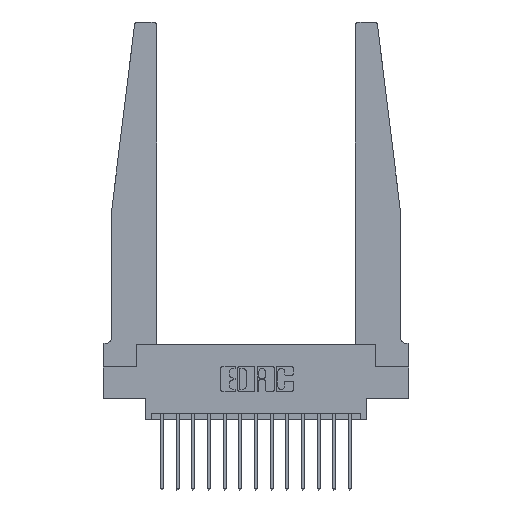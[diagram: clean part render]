
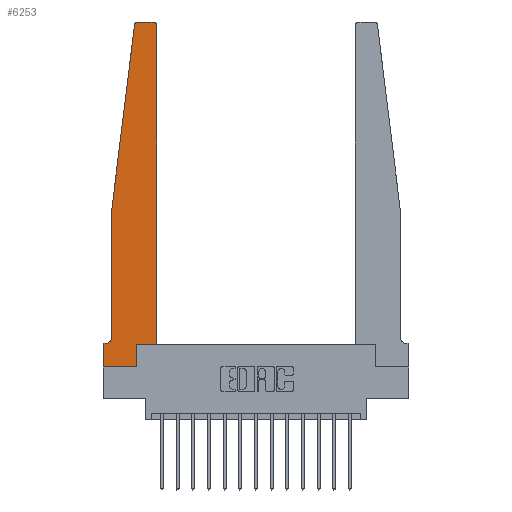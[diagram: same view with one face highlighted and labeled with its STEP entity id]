
A CAD part, top view. The second image highlights one B-rep face of the part: STEP entity #6253.
In plain terms, the highlighted planar face has unit normal (0, 0, 1).
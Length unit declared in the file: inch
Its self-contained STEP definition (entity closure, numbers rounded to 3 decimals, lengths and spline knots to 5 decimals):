
#14 = ORIENTED_EDGE ( 'NONE', *, *, #17315, .T. ) ;
#188 = LINE ( 'NONE', #2962, #15309 ) ;
#430 = CARTESIAN_POINT ( 'NONE',  ( 0.2605, 0.18, 0.37 ) ) ;
#870 = VECTOR ( 'NONE', #1512, 39.37008 ) ;
#922 = ORIENTED_EDGE ( 'NONE', *, *, #9882, .T. ) ;
#1371 = DIRECTION ( 'NONE',  ( 0., -1., 0. ) ) ;
#1512 = DIRECTION ( 'NONE',  ( 0., 1., 0. ) ) ;
#1520 = VECTOR ( 'NONE', #2605, 39.37008 ) ;
#1620 = FACE_OUTER_BOUND ( 'NONE', #4993, .T. ) ;
#2082 = CARTESIAN_POINT ( 'NONE',  ( 0.27653, 2.72, 0.37 ) ) ;
#2123 = DIRECTION ( 'NONE',  ( 0., 0., 1. ) ) ;
#2340 = VERTEX_POINT ( 'NONE', #15075 ) ;
#2605 = DIRECTION ( 'NONE',  ( 0., 1., 0. ) ) ;
#2628 = LINE ( 'NONE', #13582, #12087 ) ;
#2693 = LINE ( 'NONE', #5117, #1520 ) ;
#2732 = LINE ( 'NONE', #6477, #10902 ) ;
#2768 = VECTOR ( 'NONE', #9583, 39.37008 ) ;
#2829 = AXIS2_PLACEMENT_3D ( 'NONE', #16928, #10074, #8721 ) ;
#2962 = CARTESIAN_POINT ( 'NONE',  ( 0., 0., 0.37 ) ) ;
#2967 = DIRECTION ( 'NONE',  ( 0., 0., 1. ) ) ;
#3551 = EDGE_CURVE ( 'NONE', #14291, #2340, #7639, .T. ) ;
#3645 = ORIENTED_EDGE ( 'NONE', *, *, #12383, .T. ) ;
#3940 = ORIENTED_EDGE ( 'NONE', *, *, #3551, .T. ) ;
#4198 = LINE ( 'NONE', #430, #870 ) ;
#4570 = CARTESIAN_POINT ( 'NONE',  ( 0.24675, 2.72367, 0.37 ) ) ;
#4993 = EDGE_LOOP ( 'NONE', ( #14090, #14, #15382, #5123, #12599, #12041, #3645, #7133, #8450, #922, #17621, #3940 ) ) ;
#5117 = CARTESIAN_POINT ( 'NONE',  ( 0.425, 0.18, 0.37 ) ) ;
#5123 = ORIENTED_EDGE ( 'NONE', *, *, #12833, .T. ) ;
#5259 = VECTOR ( 'NONE', #12888, 39.37008 ) ;
#5308 = CARTESIAN_POINT ( 'NONE',  ( 0.425, 0.18, 0.37 ) ) ;
#5365 = VERTEX_POINT ( 'NONE', #8385 ) ;
#5480 = CARTESIAN_POINT ( 'NONE',  ( 0., 0.1875, 0.37 ) ) ;
#5982 = EDGE_CURVE ( 'NONE', #5365, #13628, #11136, .T. ) ;
#5983 = DIRECTION ( 'NONE',  ( -1., 0., 0. ) ) ;
#6066 = CARTESIAN_POINT ( 'NONE',  ( 0.065, 0.1875, 0.37 ) ) ;
#6074 = VERTEX_POINT ( 'NONE', #9248 ) ;
#6253 = ADVANCED_FACE ( 'NONE', ( #1620 ), #8157, .T. ) ;
#6271 = DIRECTION ( 'NONE',  ( 0., 0., 1. ) ) ;
#6477 = CARTESIAN_POINT ( 'NONE',  ( 0., 0., 0.37 ) ) ;
#6504 = AXIS2_PLACEMENT_3D ( 'NONE', #16967, #2123, #14427 ) ;
#7105 = CARTESIAN_POINT ( 'NONE',  ( 0.27653, 2.75, 0.37 ) ) ;
#7133 = ORIENTED_EDGE ( 'NONE', *, *, #14382, .T. ) ;
#7639 = CIRCLE ( 'NONE', #6504, 0.03 ) ;
#7668 = EDGE_CURVE ( 'NONE', #6074, #14740, #4198, .T. ) ;
#8157 = PLANE ( 'NONE',  #16912 ) ;
#8198 = EDGE_CURVE ( 'NONE', #13628, #11796, #8597, .T. ) ;
#8337 = CARTESIAN_POINT ( 'NONE',  ( 0.425, 2.72, 0.37 ) ) ;
#8339 = AXIS2_PLACEMENT_3D ( 'NONE', #2082, #6271, #17086 ) ;
#8385 = CARTESIAN_POINT ( 'NONE',  ( 0.065, 0.2375, 0.37 ) ) ;
#8422 = DIRECTION ( 'NONE',  ( 1., 0., 0. ) ) ;
#8450 = ORIENTED_EDGE ( 'NONE', *, *, #7668, .T. ) ;
#8541 = EDGE_CURVE ( 'NONE', #2340, #10288, #14152, .T. ) ;
#8597 = LINE ( 'NONE', #6066, #14146 ) ;
#8721 = DIRECTION ( 'NONE',  ( -1., 0., 0. ) ) ;
#8753 = CARTESIAN_POINT ( 'NONE',  ( 0.2605, 0.18, 0.37 ) ) ;
#9248 = CARTESIAN_POINT ( 'NONE',  ( 0.2605, 0., 0.37 ) ) ;
#9276 = DIRECTION ( 'NONE',  ( 0., -1., 0. ) ) ;
#9495 = VERTEX_POINT ( 'NONE', #4570 ) ;
#9583 = DIRECTION ( 'NONE',  ( 1., 0., 0. ) ) ;
#9882 = EDGE_CURVE ( 'NONE', #14740, #17104, #12373, .T. ) ;
#10074 = DIRECTION ( 'NONE',  ( 0., 0., -1. ) ) ;
#10141 = CARTESIAN_POINT ( 'NONE',  ( 0., 0.1875, 0.37 ) ) ;
#10253 = VERTEX_POINT ( 'NONE', #15503 ) ;
#10288 = VERTEX_POINT ( 'NONE', #7105 ) ;
#10773 = LINE ( 'NONE', #13397, #15845 ) ;
#10902 = VECTOR ( 'NONE', #9276, 39.37008 ) ;
#10948 = DIRECTION ( 'NONE',  ( 1., 0., 0. ) ) ;
#11136 = CIRCLE ( 'NONE', #2829, 0.05 ) ;
#11796 = VERTEX_POINT ( 'NONE', #10141 ) ;
#12041 = ORIENTED_EDGE ( 'NONE', *, *, #8198, .T. ) ;
#12087 = VECTOR ( 'NONE', #1371, 39.37008 ) ;
#12373 = LINE ( 'NONE', #12458, #2768 ) ;
#12383 = EDGE_CURVE ( 'NONE', #11796, #10253, #2732, .T. ) ;
#12458 = CARTESIAN_POINT ( 'NONE',  ( 0.425, 0.18, 0.37 ) ) ;
#12599 = ORIENTED_EDGE ( 'NONE', *, *, #5982, .T. ) ;
#12833 = EDGE_CURVE ( 'NONE', #14110, #5365, #2628, .T. ) ;
#12834 = EDGE_CURVE ( 'NONE', #9495, #14110, #10773, .T. ) ;
#12888 = DIRECTION ( 'NONE',  ( -1., 0., 0. ) ) ;
#13397 = CARTESIAN_POINT ( 'NONE',  ( 0.065, 1.25, 0.37 ) ) ;
#13494 = DIRECTION ( 'NONE',  ( -0.122, -0.992, 0. ) ) ;
#13582 = CARTESIAN_POINT ( 'NONE',  ( 0.065, 1.25, 0.37 ) ) ;
#13628 = VERTEX_POINT ( 'NONE', #14336 ) ;
#14090 = ORIENTED_EDGE ( 'NONE', *, *, #8541, .T. ) ;
#14110 = VERTEX_POINT ( 'NONE', #15016 ) ;
#14135 = EDGE_CURVE ( 'NONE', #17104, #14291, #2693, .T. ) ;
#14146 = VECTOR ( 'NONE', #5983, 39.37008 ) ;
#14152 = LINE ( 'NONE', #15518, #5259 ) ;
#14291 = VERTEX_POINT ( 'NONE', #8337 ) ;
#14336 = CARTESIAN_POINT ( 'NONE',  ( 0.015, 0.1875, 0.37 ) ) ;
#14382 = EDGE_CURVE ( 'NONE', #10253, #6074, #188, .T. ) ;
#14427 = DIRECTION ( 'NONE',  ( 1., 0., 0. ) ) ;
#14740 = VERTEX_POINT ( 'NONE', #8753 ) ;
#15016 = CARTESIAN_POINT ( 'NONE',  ( 0.065, 1.25, 0.37 ) ) ;
#15075 = CARTESIAN_POINT ( 'NONE',  ( 0.395, 2.75, 0.37 ) ) ;
#15309 = VECTOR ( 'NONE', #8422, 39.37008 ) ;
#15382 = ORIENTED_EDGE ( 'NONE', *, *, #12834, .T. ) ;
#15503 = CARTESIAN_POINT ( 'NONE',  ( 0., 0., 0.37 ) ) ;
#15518 = CARTESIAN_POINT ( 'NONE',  ( 0.25, 2.75, 0.37 ) ) ;
#15845 = VECTOR ( 'NONE', #13494, 39.37008 ) ;
#16395 = CIRCLE ( 'NONE', #8339, 0.03 ) ;
#16912 = AXIS2_PLACEMENT_3D ( 'NONE', #5480, #2967, #10948 ) ;
#16928 = CARTESIAN_POINT ( 'NONE',  ( 0.015, 0.2375, 0.37 ) ) ;
#16967 = CARTESIAN_POINT ( 'NONE',  ( 0.395, 2.72, 0.37 ) ) ;
#17086 = DIRECTION ( 'NONE',  ( 1., 0., 0. ) ) ;
#17104 = VERTEX_POINT ( 'NONE', #5308 ) ;
#17315 = EDGE_CURVE ( 'NONE', #10288, #9495, #16395, .T. ) ;
#17621 = ORIENTED_EDGE ( 'NONE', *, *, #14135, .T. ) ;
